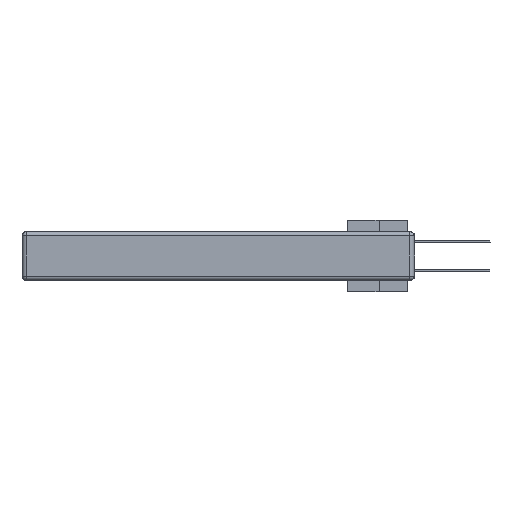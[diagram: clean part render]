
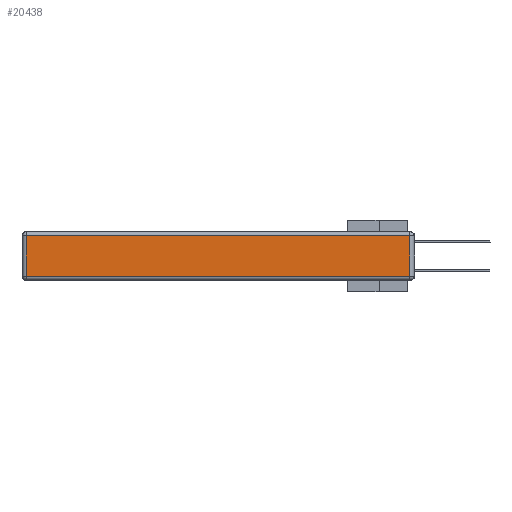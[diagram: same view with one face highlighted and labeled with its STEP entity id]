
A CAD part, left-side view. The second image highlights one B-rep face of the part: STEP entity #20438.
In plain terms, the highlighted planar face has unit normal (-1, 0, 0).
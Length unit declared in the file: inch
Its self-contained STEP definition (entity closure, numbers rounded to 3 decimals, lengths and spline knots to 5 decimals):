
#2440 = DIRECTION ( 'NONE',  ( 0., 0., 1. ) ) ;
#2610 = CARTESIAN_POINT ( 'NONE',  ( 0., 2.72, -0.03 ) ) ;
#3320 = EDGE_CURVE ( 'NONE', #16045, #8313, #26363, .T. ) ;
#3494 = VECTOR ( 'NONE', #20456, 39.37008 ) ;
#4770 = ORIENTED_EDGE ( 'NONE', *, *, #15428, .T. ) ;
#4846 = LINE ( 'NONE', #11920, #22075 ) ;
#6076 = CARTESIAN_POINT ( 'NONE',  ( 0., 2.72, -0.313 ) ) ;
#7295 = CARTESIAN_POINT ( 'NONE',  ( 0., 0., -0.343 ) ) ;
#7458 = LINE ( 'NONE', #23288, #3494 ) ;
#8313 = VERTEX_POINT ( 'NONE', #2610 ) ;
#8415 = VECTOR ( 'NONE', #2440, 39.37008 ) ;
#8924 = CARTESIAN_POINT ( 'NONE',  ( 0., 0.03, -0.313 ) ) ;
#9684 = EDGE_CURVE ( 'NONE', #19546, #16045, #15053, .T. ) ;
#11225 = ORIENTED_EDGE ( 'NONE', *, *, #13705, .T. ) ;
#11920 = CARTESIAN_POINT ( 'NONE',  ( 0., 0., -0.313 ) ) ;
#13032 = VECTOR ( 'NONE', #21667, 39.37008 ) ;
#13705 = EDGE_CURVE ( 'NONE', #26447, #19546, #4846, .T. ) ;
#15053 = LINE ( 'NONE', #20290, #8415 ) ;
#15428 = EDGE_CURVE ( 'NONE', #8313, #26447, #7458, .T. ) ;
#16045 = VERTEX_POINT ( 'NONE', #20084 ) ;
#16428 = DIRECTION ( 'NONE',  ( 0., 0., 1. ) ) ;
#19546 = VERTEX_POINT ( 'NONE', #8924 ) ;
#20084 = CARTESIAN_POINT ( 'NONE',  ( 0., 0.03, -0.03 ) ) ;
#20230 = FACE_OUTER_BOUND ( 'NONE', #25908, .T. ) ;
#20290 = CARTESIAN_POINT ( 'NONE',  ( 0., 0.03, -0.343 ) ) ;
#20438 = ADVANCED_FACE ( 'NONE', ( #20230 ), #32003, .T. ) ;
#20456 = DIRECTION ( 'NONE',  ( 0., 0., -1. ) ) ;
#21667 = DIRECTION ( 'NONE',  ( 0., 1., 0. ) ) ;
#22075 = VECTOR ( 'NONE', #32187, 39.37008 ) ;
#23288 = CARTESIAN_POINT ( 'NONE',  ( 0., 2.72, -0.343 ) ) ;
#23364 = DIRECTION ( 'NONE',  ( -1., 0., 0. ) ) ;
#25908 = EDGE_LOOP ( 'NONE', ( #11225, #31094, #29067, #4770 ) ) ;
#26018 = AXIS2_PLACEMENT_3D ( 'NONE', #7295, #23364, #16428 ) ;
#26363 = LINE ( 'NONE', #26384, #13032 ) ;
#26384 = CARTESIAN_POINT ( 'NONE',  ( 0., 2.75, -0.03 ) ) ;
#26447 = VERTEX_POINT ( 'NONE', #6076 ) ;
#29067 = ORIENTED_EDGE ( 'NONE', *, *, #3320, .T. ) ;
#31094 = ORIENTED_EDGE ( 'NONE', *, *, #9684, .T. ) ;
#32003 = PLANE ( 'NONE',  #26018 ) ;
#32187 = DIRECTION ( 'NONE',  ( 0., -1., 0. ) ) ;
